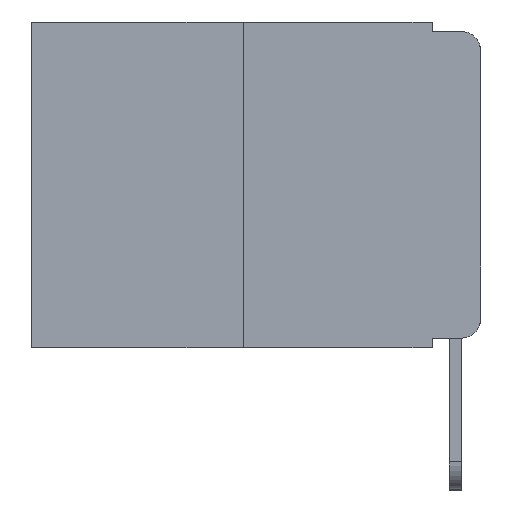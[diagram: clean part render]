
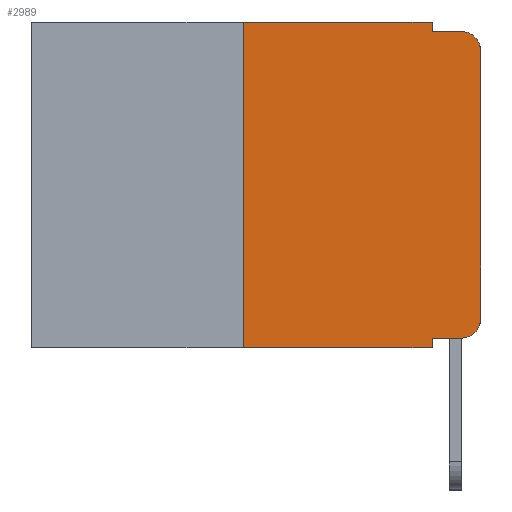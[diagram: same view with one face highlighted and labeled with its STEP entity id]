
A CAD part, left-side view. The second image highlights one B-rep face of the part: STEP entity #2989.
In plain terms, the highlighted planar face has unit normal (-1, 0, 0).
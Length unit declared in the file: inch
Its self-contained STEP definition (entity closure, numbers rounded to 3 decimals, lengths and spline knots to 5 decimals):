
#460 = AXIS2_PLACEMENT_3D ( 'NONE', #10601, #6041, #10787 ) ;
#921 = DIRECTION ( 'NONE',  ( 0., 0., 1. ) ) ;
#1115 = VERTEX_POINT ( 'NONE', #2927 ) ;
#1437 = VERTEX_POINT ( 'NONE', #5544 ) ;
#1708 = LINE ( 'NONE', #4178, #10374 ) ;
#1758 = CARTESIAN_POINT ( 'NONE',  ( 0., 0.25, -0.343 ) ) ;
#2228 = ORIENTED_EDGE ( 'NONE', *, *, #2649, .T. ) ;
#2327 = ORIENTED_EDGE ( 'NONE', *, *, #10059, .F. ) ;
#2419 = ORIENTED_EDGE ( 'NONE', *, *, #10663, .T. ) ;
#2649 = EDGE_CURVE ( 'NONE', #9269, #6362, #9909, .T. ) ;
#2729 = ORIENTED_EDGE ( 'NONE', *, *, #11135, .T. ) ;
#2741 = ORIENTED_EDGE ( 'NONE', *, *, #7522, .F. ) ;
#2833 = ORIENTED_EDGE ( 'NONE', *, *, #10236, .F. ) ;
#2927 = CARTESIAN_POINT ( 'NONE',  ( 0., 0.25, 0. ) ) ;
#2989 = ADVANCED_FACE ( 'NONE', ( #9682 ), #3403, .F. ) ;
#3018 = CARTESIAN_POINT ( 'NONE',  ( 0., 0., 0. ) ) ;
#3112 = VERTEX_POINT ( 'NONE', #8606 ) ;
#3138 = ORIENTED_EDGE ( 'NONE', *, *, #10472, .F. ) ;
#3209 = ORIENTED_EDGE ( 'NONE', *, *, #8889, .T. ) ;
#3403 = PLANE ( 'NONE',  #3984 ) ;
#3688 = CARTESIAN_POINT ( 'NONE',  ( 0., 0.051, -0.01 ) ) ;
#3713 = ORIENTED_EDGE ( 'NONE', *, *, #8832, .T. ) ;
#3811 = DIRECTION ( 'NONE',  ( 0., -1., 0. ) ) ;
#3984 = AXIS2_PLACEMENT_3D ( 'NONE', #11076, #10167, #9372 ) ;
#4119 = DIRECTION ( 'NONE',  ( 0., 0., 1. ) ) ;
#4178 = CARTESIAN_POINT ( 'NONE',  ( 0., 0.25, 0. ) ) ;
#4236 = ORIENTED_EDGE ( 'NONE', *, *, #10075, .F. ) ;
#4256 = LINE ( 'NONE', #5984, #6323 ) ;
#4278 = CARTESIAN_POINT ( 'NONE',  ( 0., 0.473, -0.343 ) ) ;
#4411 = VERTEX_POINT ( 'NONE', #6511 ) ;
#4476 = VECTOR ( 'NONE', #8563, 39.37008 ) ;
#4705 = DIRECTION ( 'NONE',  ( 0., -1., 0. ) ) ;
#4783 = LINE ( 'NONE', #6281, #4476 ) ;
#5476 = VERTEX_POINT ( 'NONE', #6831 ) ;
#5508 = VERTEX_POINT ( 'NONE', #10692 ) ;
#5544 = CARTESIAN_POINT ( 'NONE',  ( 0., 0.02, -0.333 ) ) ;
#5573 = LINE ( 'NONE', #9987, #6905 ) ;
#5847 = CIRCLE ( 'NONE', #460, 0.02 ) ;
#5942 = DIRECTION ( 'NONE',  ( -1., 0., 0. ) ) ;
#5984 = CARTESIAN_POINT ( 'NONE',  ( 0., 0.051, 0. ) ) ;
#6041 = DIRECTION ( 'NONE',  ( -1., 0., 0. ) ) ;
#6079 = CARTESIAN_POINT ( 'NONE',  ( 0., 0.051, -0.343 ) ) ;
#6151 = DIRECTION ( 'NONE',  ( 0., 0., -1. ) ) ;
#6281 = CARTESIAN_POINT ( 'NONE',  ( 0., 0.473, 0. ) ) ;
#6323 = VECTOR ( 'NONE', #10519, 39.37008 ) ;
#6362 = VERTEX_POINT ( 'NONE', #6079 ) ;
#6511 = CARTESIAN_POINT ( 'NONE',  ( 0., 0., -0.03 ) ) ;
#6663 = AXIS2_PLACEMENT_3D ( 'NONE', #10505, #5942, #11209 ) ;
#6788 = LINE ( 'NONE', #3688, #10598 ) ;
#6831 = CARTESIAN_POINT ( 'NONE',  ( 0., 0.051, 0. ) ) ;
#6905 = VECTOR ( 'NONE', #6151, 39.37008 ) ;
#7522 = EDGE_CURVE ( 'NONE', #1115, #5476, #4783, .T. ) ;
#7871 = VECTOR ( 'NONE', #9320, 39.37008 ) ;
#8128 = EDGE_LOOP ( 'NONE', ( #3713, #3209, #3138, #2833, #2741, #2327, #2228, #4236, #2729, #2419 ) ) ;
#8435 = VECTOR ( 'NONE', #3811, 39.37008 ) ;
#8563 = DIRECTION ( 'NONE',  ( 0., -1., 0. ) ) ;
#8606 = CARTESIAN_POINT ( 'NONE',  ( 0., 0.051, -0.333 ) ) ;
#8607 = VECTOR ( 'NONE', #4119, 39.37008 ) ;
#8684 = LINE ( 'NONE', #11004, #8435 ) ;
#8832 = EDGE_CURVE ( 'NONE', #5508, #4411, #10398, .T. ) ;
#8889 = EDGE_CURVE ( 'NONE', #4411, #9444, #5847, .T. ) ;
#9052 = CARTESIAN_POINT ( 'NONE',  ( 0., 0.02, -0.01 ) ) ;
#9269 = VERTEX_POINT ( 'NONE', #1758 ) ;
#9320 = DIRECTION ( 'NONE',  ( 0., -1., 0. ) ) ;
#9372 = DIRECTION ( 'NONE',  ( 0., 0., -1. ) ) ;
#9444 = VERTEX_POINT ( 'NONE', #9052 ) ;
#9682 = FACE_OUTER_BOUND ( 'NONE', #8128, .T. ) ;
#9909 = LINE ( 'NONE', #4278, #7871 ) ;
#9987 = CARTESIAN_POINT ( 'NONE',  ( 0., 0.051, 0. ) ) ;
#10042 = CARTESIAN_POINT ( 'NONE',  ( 0., 0.051, -0.01 ) ) ;
#10059 = EDGE_CURVE ( 'NONE', #9269, #1115, #1708, .T. ) ;
#10075 = EDGE_CURVE ( 'NONE', #3112, #6362, #4256, .T. ) ;
#10167 = DIRECTION ( 'NONE',  ( 1., 0., 0. ) ) ;
#10236 = EDGE_CURVE ( 'NONE', #5476, #10862, #5573, .T. ) ;
#10374 = VECTOR ( 'NONE', #921, 39.37008 ) ;
#10398 = LINE ( 'NONE', #3018, #8607 ) ;
#10472 = EDGE_CURVE ( 'NONE', #10862, #9444, #6788, .T. ) ;
#10505 = CARTESIAN_POINT ( 'NONE',  ( 0., 0.02, -0.313 ) ) ;
#10519 = DIRECTION ( 'NONE',  ( 0., 0., -1. ) ) ;
#10598 = VECTOR ( 'NONE', #4705, 39.37008 ) ;
#10601 = CARTESIAN_POINT ( 'NONE',  ( 0., 0.02, -0.03 ) ) ;
#10663 = EDGE_CURVE ( 'NONE', #1437, #5508, #10709, .T. ) ;
#10692 = CARTESIAN_POINT ( 'NONE',  ( 0., 0., -0.313 ) ) ;
#10709 = CIRCLE ( 'NONE', #6663, 0.02 ) ;
#10787 = DIRECTION ( 'NONE',  ( 0., 0., -1. ) ) ;
#10862 = VERTEX_POINT ( 'NONE', #10042 ) ;
#11004 = CARTESIAN_POINT ( 'NONE',  ( 0., 0.051, -0.333 ) ) ;
#11076 = CARTESIAN_POINT ( 'NONE',  ( 0., 0.473, 0. ) ) ;
#11135 = EDGE_CURVE ( 'NONE', #3112, #1437, #8684, .T. ) ;
#11209 = DIRECTION ( 'NONE',  ( 0., 0., -1. ) ) ;
